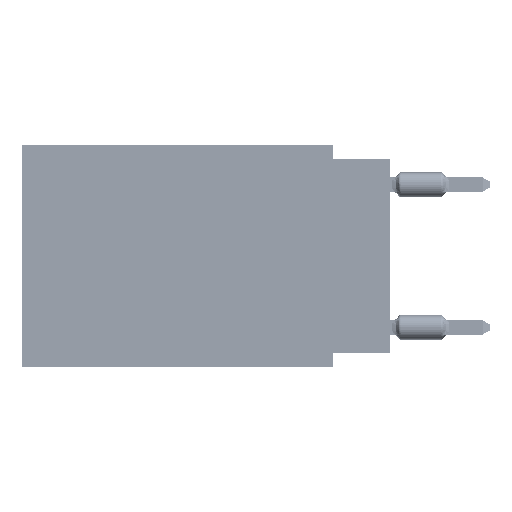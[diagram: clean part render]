
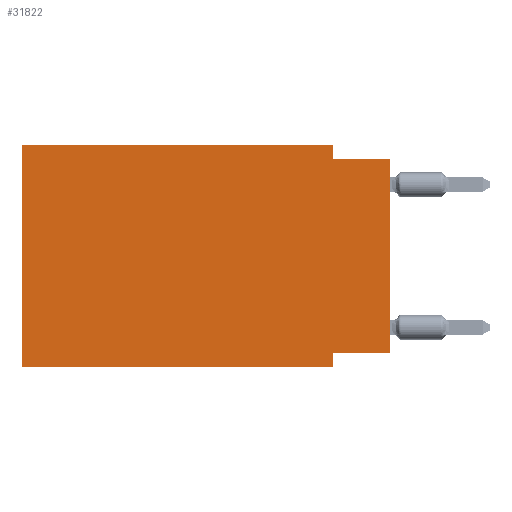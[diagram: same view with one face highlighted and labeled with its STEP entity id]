
A CAD part, left-side view. The second image highlights one B-rep face of the part: STEP entity #31822.
In plain terms, the highlighted planar face has unit normal (-1, 0, 0).
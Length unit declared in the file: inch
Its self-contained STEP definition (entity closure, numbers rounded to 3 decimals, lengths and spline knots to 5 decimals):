
#53 = DIRECTION ( 'NONE',  ( 0., 0., -1. ) ) ;
#1971 = CARTESIAN_POINT ( 'NONE',  ( 0., 0.1, -0.39 ) ) ;
#2859 = VECTOR ( 'NONE', #31769, 39.37008 ) ;
#3059 = VERTEX_POINT ( 'NONE', #1971 ) ;
#4000 = ORIENTED_EDGE ( 'NONE', *, *, #52786, .F. ) ;
#4568 = CARTESIAN_POINT ( 'NONE',  ( 0., 0.645, 0. ) ) ;
#6013 = LINE ( 'NONE', #39829, #46906 ) ;
#6947 = CARTESIAN_POINT ( 'NONE',  ( 0., 0., -0.025 ) ) ;
#7825 = LINE ( 'NONE', #12426, #2859 ) ;
#10467 = CARTESIAN_POINT ( 'NONE',  ( 0., 0.1, -0.39 ) ) ;
#10701 = VERTEX_POINT ( 'NONE', #32827 ) ;
#12426 = CARTESIAN_POINT ( 'NONE',  ( 0., 0.1, 0. ) ) ;
#14387 = LINE ( 'NONE', #51942, #30567 ) ;
#15567 = DIRECTION ( 'NONE',  ( 0., 0., 1. ) ) ;
#16017 = EDGE_CURVE ( 'NONE', #33904, #3059, #52611, .T. ) ;
#16123 = DIRECTION ( 'NONE',  ( 0., -1., 0. ) ) ;
#18111 = VECTOR ( 'NONE', #53, 39.37008 ) ;
#18546 = ORIENTED_EDGE ( 'NONE', *, *, #57576, .F. ) ;
#18708 = LINE ( 'NONE', #28272, #38453 ) ;
#18747 = DIRECTION ( 'NONE',  ( 1., 0., 0. ) ) ;
#19241 = AXIS2_PLACEMENT_3D ( 'NONE', #42166, #18747, #34713 ) ;
#19563 = ORIENTED_EDGE ( 'NONE', *, *, #16017, .F. ) ;
#23083 = ORIENTED_EDGE ( 'NONE', *, *, #39163, .T. ) ;
#23201 = EDGE_CURVE ( 'NONE', #25764, #55037, #6013, .T. ) ;
#23390 = PLANE ( 'NONE',  #19241 ) ;
#23943 = DIRECTION ( 'NONE',  ( 0., 1., 0. ) ) ;
#25040 = VERTEX_POINT ( 'NONE', #44523 ) ;
#25764 = VERTEX_POINT ( 'NONE', #27041 ) ;
#27041 = CARTESIAN_POINT ( 'NONE',  ( 0., 0.1, -0.025 ) ) ;
#27528 = VECTOR ( 'NONE', #39284, 39.37008 ) ;
#27669 = VECTOR ( 'NONE', #15567, 39.37008 ) ;
#28272 = CARTESIAN_POINT ( 'NONE',  ( 0., 0., -0.365 ) ) ;
#28299 = VECTOR ( 'NONE', #46275, 39.37008 ) ;
#28616 = EDGE_CURVE ( 'NONE', #10701, #33904, #18708, .T. ) ;
#28706 = ORIENTED_EDGE ( 'NONE', *, *, #23201, .F. ) ;
#29410 = LINE ( 'NONE', #47572, #27669 ) ;
#29725 = CARTESIAN_POINT ( 'NONE',  ( 0., 0.645, 0. ) ) ;
#30567 = VECTOR ( 'NONE', #43294, 39.37008 ) ;
#31769 = DIRECTION ( 'NONE',  ( 0., 0., -1. ) ) ;
#31822 = ADVANCED_FACE ( 'NONE', ( #46778 ), #23390, .F. ) ;
#32391 = CARTESIAN_POINT ( 'NONE',  ( 0., 0.645, 0. ) ) ;
#32827 = CARTESIAN_POINT ( 'NONE',  ( 0., 0., -0.365 ) ) ;
#33861 = CARTESIAN_POINT ( 'NONE',  ( 0., 0.1, 0. ) ) ;
#33904 = VERTEX_POINT ( 'NONE', #48148 ) ;
#34713 = DIRECTION ( 'NONE',  ( 0., 0., -1. ) ) ;
#37720 = ORIENTED_EDGE ( 'NONE', *, *, #54130, .F. ) ;
#38453 = VECTOR ( 'NONE', #23943, 39.37008 ) ;
#39163 = EDGE_CURVE ( 'NONE', #10701, #55037, #29410, .T. ) ;
#39284 = DIRECTION ( 'NONE',  ( 0., 0., 1. ) ) ;
#39703 = EDGE_LOOP ( 'NONE', ( #23083, #28706, #37720, #4000, #18546, #39917, #19563, #41634 ) ) ;
#39829 = CARTESIAN_POINT ( 'NONE',  ( 0., 0., -0.025 ) ) ;
#39917 = ORIENTED_EDGE ( 'NONE', *, *, #45635, .T. ) ;
#41142 = VERTEX_POINT ( 'NONE', #33861 ) ;
#41634 = ORIENTED_EDGE ( 'NONE', *, *, #28616, .F. ) ;
#42166 = CARTESIAN_POINT ( 'NONE',  ( 0., 0.645, 0. ) ) ;
#43294 = DIRECTION ( 'NONE',  ( 0., -1., 0. ) ) ;
#44503 = LINE ( 'NONE', #29725, #27528 ) ;
#44523 = CARTESIAN_POINT ( 'NONE',  ( 0., 0.645, -0.39 ) ) ;
#45635 = EDGE_CURVE ( 'NONE', #25040, #3059, #14387, .T. ) ;
#46275 = DIRECTION ( 'NONE',  ( 0., -1., 0. ) ) ;
#46778 = FACE_OUTER_BOUND ( 'NONE', #39703, .T. ) ;
#46906 = VECTOR ( 'NONE', #16123, 39.37008 ) ;
#47572 = CARTESIAN_POINT ( 'NONE',  ( 0., 0., 0. ) ) ;
#48148 = CARTESIAN_POINT ( 'NONE',  ( 0., 0.1, -0.365 ) ) ;
#51942 = CARTESIAN_POINT ( 'NONE',  ( 0., 0.645, -0.39 ) ) ;
#52611 = LINE ( 'NONE', #10467, #18111 ) ;
#52786 = EDGE_CURVE ( 'NONE', #57323, #41142, #59811, .T. ) ;
#54130 = EDGE_CURVE ( 'NONE', #41142, #25764, #7825, .T. ) ;
#55037 = VERTEX_POINT ( 'NONE', #6947 ) ;
#57323 = VERTEX_POINT ( 'NONE', #4568 ) ;
#57576 = EDGE_CURVE ( 'NONE', #25040, #57323, #44503, .T. ) ;
#59811 = LINE ( 'NONE', #32391, #28299 ) ;
